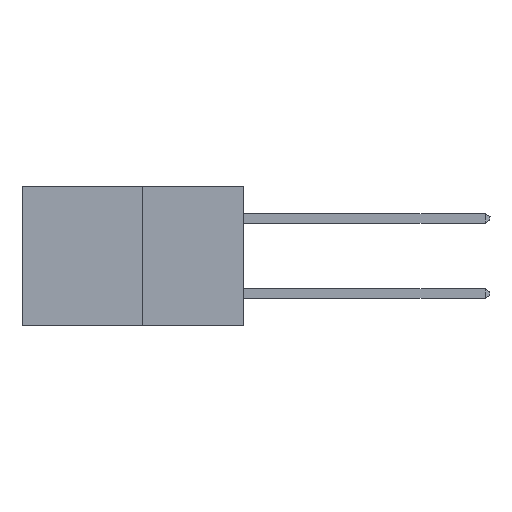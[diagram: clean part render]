
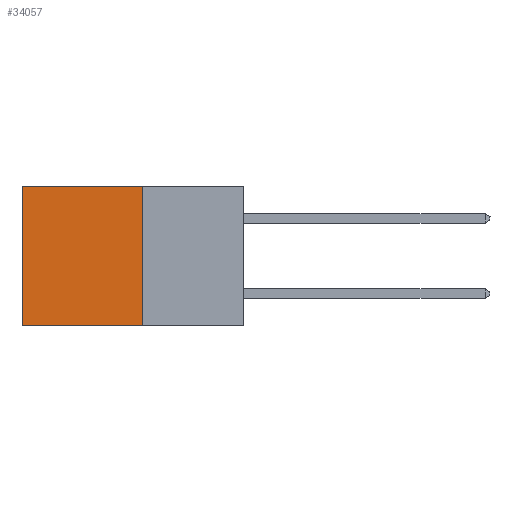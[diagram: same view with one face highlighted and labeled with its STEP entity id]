
A CAD part, left-side view. The second image highlights one B-rep face of the part: STEP entity #34057.
In plain terms, the highlighted planar face has unit normal (-1, 0, 0).
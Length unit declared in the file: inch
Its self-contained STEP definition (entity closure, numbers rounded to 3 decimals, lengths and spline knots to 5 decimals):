
#84 = VERTEX_POINT ( 'NONE', #29924 ) ;
#1043 = ORIENTED_EDGE ( 'NONE', *, *, #26301, .T. ) ;
#1054 = EDGE_CURVE ( 'NONE', #84, #19204, #31016, .T. ) ;
#1092 = VERTEX_POINT ( 'NONE', #12464 ) ;
#1314 = DIRECTION ( 'NONE',  ( 0., 0., -1. ) ) ;
#2863 = VECTOR ( 'NONE', #31461, 39.37008 ) ;
#3840 = EDGE_LOOP ( 'NONE', ( #1043, #20053, #27837, #19690 ) ) ;
#7634 = LINE ( 'NONE', #19193, #20903 ) ;
#8002 = CARTESIAN_POINT ( 'NONE',  ( 0.277, 0.59, -0.37 ) ) ;
#8872 = AXIS2_PLACEMENT_3D ( 'NONE', #11994, #33019, #17339 ) ;
#9278 = PLANE ( 'NONE',  #8872 ) ;
#11994 = CARTESIAN_POINT ( 'NONE',  ( 0.277, 0.27, -0.37 ) ) ;
#12464 = CARTESIAN_POINT ( 'NONE',  ( 0.277, 0.27, -0.37 ) ) ;
#13491 = DIRECTION ( 'NONE',  ( 0., 0., -1. ) ) ;
#14993 = LINE ( 'NONE', #21460, #34249 ) ;
#15729 = CARTESIAN_POINT ( 'NONE',  ( 0.277, 0.59, 0. ) ) ;
#17317 = CARTESIAN_POINT ( 'NONE',  ( 0.277, 0.27, -0.37 ) ) ;
#17339 = DIRECTION ( 'NONE',  ( 0., 0., -1. ) ) ;
#17444 = EDGE_CURVE ( 'NONE', #84, #1092, #33971, .T. ) ;
#19193 = CARTESIAN_POINT ( 'NONE',  ( 0.277, 0.27, -0.37 ) ) ;
#19204 = VERTEX_POINT ( 'NONE', #15729 ) ;
#19690 = ORIENTED_EDGE ( 'NONE', *, *, #1054, .T. ) ;
#20053 = ORIENTED_EDGE ( 'NONE', *, *, #33831, .F. ) ;
#20903 = VECTOR ( 'NONE', #21835, 39.37008 ) ;
#21306 = FACE_OUTER_BOUND ( 'NONE', #3840, .T. ) ;
#21460 = CARTESIAN_POINT ( 'NONE',  ( 0.277, 0.59, -0.37 ) ) ;
#21835 = DIRECTION ( 'NONE',  ( 0., 1., 0. ) ) ;
#26235 = VERTEX_POINT ( 'NONE', #8002 ) ;
#26301 = EDGE_CURVE ( 'NONE', #19204, #26235, #14993, .T. ) ;
#27834 = CARTESIAN_POINT ( 'NONE',  ( 0.277, 0.27, 0. ) ) ;
#27837 = ORIENTED_EDGE ( 'NONE', *, *, #17444, .F. ) ;
#29924 = CARTESIAN_POINT ( 'NONE',  ( 0.277, 0.27, 0. ) ) ;
#31016 = LINE ( 'NONE', #27834, #2863 ) ;
#31461 = DIRECTION ( 'NONE',  ( 0., 1., 0. ) ) ;
#32331 = VECTOR ( 'NONE', #1314, 39.37008 ) ;
#33019 = DIRECTION ( 'NONE',  ( 1., 0., 0. ) ) ;
#33831 = EDGE_CURVE ( 'NONE', #1092, #26235, #7634, .T. ) ;
#33971 = LINE ( 'NONE', #17317, #32331 ) ;
#34057 = ADVANCED_FACE ( 'NONE', ( #21306 ), #9278, .F. ) ;
#34249 = VECTOR ( 'NONE', #13491, 39.37008 ) ;
